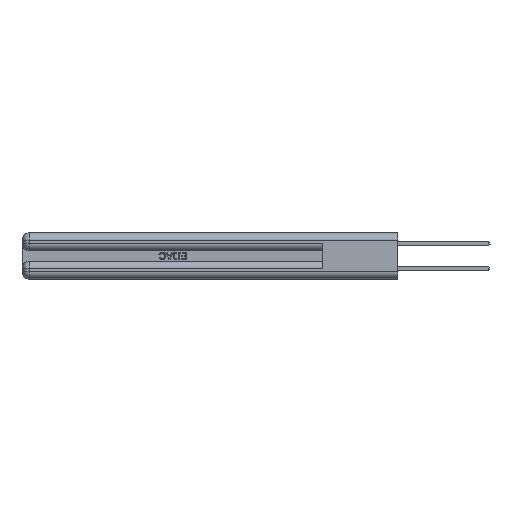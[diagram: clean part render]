
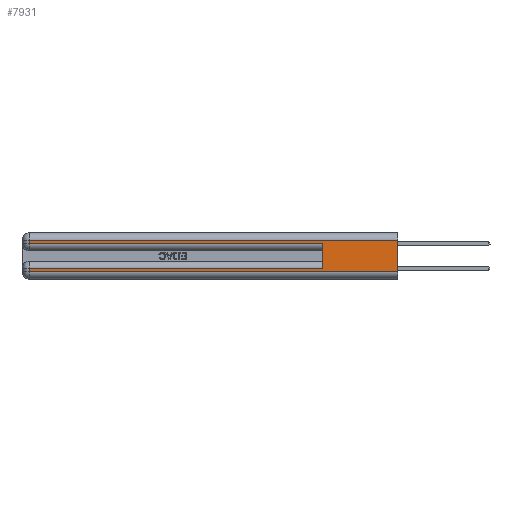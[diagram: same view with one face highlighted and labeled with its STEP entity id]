
A CAD part, left-side view. The second image highlights one B-rep face of the part: STEP entity #7931.
In plain terms, the highlighted planar face has unit normal (-1, 0, 0).
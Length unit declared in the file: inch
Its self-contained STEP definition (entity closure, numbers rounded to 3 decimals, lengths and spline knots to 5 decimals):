
#807 = ORIENTED_EDGE ( 'NONE', *, *, #41067, .T. ) ;
#837 = EDGE_CURVE ( 'NONE', #49698, #30197, #3433, .T. ) ;
#1463 = EDGE_CURVE ( 'NONE', #36310, #22740, #43413, .T. ) ;
#1693 = LINE ( 'NONE', #10921, #42359 ) ;
#2416 = DIRECTION ( 'NONE',  ( 0., -1., 0. ) ) ;
#3433 = LINE ( 'NONE', #16489, #44101 ) ;
#4040 = DIRECTION ( 'NONE',  ( 0., 0., -1. ) ) ;
#4311 = LINE ( 'NONE', #28786, #36922 ) ;
#4662 = AXIS2_PLACEMENT_3D ( 'NONE', #22745, #7198, #34738 ) ;
#4746 = ORIENTED_EDGE ( 'NONE', *, *, #12398, .T. ) ;
#4792 = VERTEX_POINT ( 'NONE', #29184 ) ;
#5282 = DIRECTION ( 'NONE',  ( 0., -1., 0. ) ) ;
#5561 = LINE ( 'NONE', #48295, #34497 ) ;
#7198 = DIRECTION ( 'NONE',  ( 1., 0., 0. ) ) ;
#7931 = ADVANCED_FACE ( 'NONE', ( #9622 ), #30686, .F. ) ;
#8285 = CARTESIAN_POINT ( 'NONE',  ( 0., 0., 0.31 ) ) ;
#9622 = FACE_OUTER_BOUND ( 'NONE', #47696, .T. ) ;
#9890 = CARTESIAN_POINT ( 'NONE',  ( 0., 2.94, 0.285 ) ) ;
#10921 = CARTESIAN_POINT ( 'NONE',  ( 0., 0., 0.37 ) ) ;
#11532 = CARTESIAN_POINT ( 'NONE',  ( 0., 2.94, 0.085 ) ) ;
#11778 = CARTESIAN_POINT ( 'NONE',  ( 0., 2.94, 0.37 ) ) ;
#12398 = EDGE_CURVE ( 'NONE', #28507, #34046, #4311, .T. ) ;
#12491 = CARTESIAN_POINT ( 'NONE',  ( 0., 0.6, 0.145 ) ) ;
#12854 = DIRECTION ( 'NONE',  ( 0., 1., 0. ) ) ;
#16391 = DIRECTION ( 'NONE',  ( 0., 0., 1. ) ) ;
#16489 = CARTESIAN_POINT ( 'NONE',  ( 0., 0., 0.085 ) ) ;
#16516 = VECTOR ( 'NONE', #4040, 39.37008 ) ;
#20144 = ORIENTED_EDGE ( 'NONE', *, *, #837, .T. ) ;
#22740 = VERTEX_POINT ( 'NONE', #41359 ) ;
#22745 = CARTESIAN_POINT ( 'NONE',  ( 0., 0., 0.37 ) ) ;
#23728 = CARTESIAN_POINT ( 'NONE',  ( 0., 0.6, 0.085 ) ) ;
#23778 = ORIENTED_EDGE ( 'NONE', *, *, #37049, .F. ) ;
#25498 = LINE ( 'NONE', #12491, #45324 ) ;
#26975 = LINE ( 'NONE', #11778, #16516 ) ;
#27406 = EDGE_CURVE ( 'NONE', #31264, #4792, #47996, .T. ) ;
#28231 = EDGE_CURVE ( 'NONE', #36310, #34046, #1693, .T. ) ;
#28459 = CARTESIAN_POINT ( 'NONE',  ( 0., 0., 0.31 ) ) ;
#28507 = VERTEX_POINT ( 'NONE', #28527 ) ;
#28527 = CARTESIAN_POINT ( 'NONE',  ( 0., 2.94, 0.06 ) ) ;
#28786 = CARTESIAN_POINT ( 'NONE',  ( 0., 0., 0.06 ) ) ;
#28902 = ORIENTED_EDGE ( 'NONE', *, *, #42451, .T. ) ;
#29184 = CARTESIAN_POINT ( 'NONE',  ( 0., 0.6, 0.285 ) ) ;
#30197 = VERTEX_POINT ( 'NONE', #11532 ) ;
#30293 = ORIENTED_EDGE ( 'NONE', *, *, #28231, .F. ) ;
#30686 = PLANE ( 'NONE',  #4662 ) ;
#31264 = VERTEX_POINT ( 'NONE', #9890 ) ;
#32852 = VECTOR ( 'NONE', #12854, 39.37008 ) ;
#33701 = CARTESIAN_POINT ( 'NONE',  ( 0., 0., 0.06 ) ) ;
#34046 = VERTEX_POINT ( 'NONE', #33701 ) ;
#34497 = VECTOR ( 'NONE', #44167, 39.37008 ) ;
#34738 = DIRECTION ( 'NONE',  ( 0., 0., -1. ) ) ;
#35167 = ORIENTED_EDGE ( 'NONE', *, *, #27406, .T. ) ;
#36310 = VERTEX_POINT ( 'NONE', #8285 ) ;
#36922 = VECTOR ( 'NONE', #5282, 39.37008 ) ;
#37049 = EDGE_CURVE ( 'NONE', #49698, #4792, #25498, .T. ) ;
#37647 = CARTESIAN_POINT ( 'NONE',  ( 0., 0., 0.285 ) ) ;
#40161 = DIRECTION ( 'NONE',  ( 0., 1., 0. ) ) ;
#41067 = EDGE_CURVE ( 'NONE', #30197, #28507, #5561, .T. ) ;
#41359 = CARTESIAN_POINT ( 'NONE',  ( 0., 2.94, 0.31 ) ) ;
#42359 = VECTOR ( 'NONE', #50333, 39.37008 ) ;
#42451 = EDGE_CURVE ( 'NONE', #22740, #31264, #26975, .T. ) ;
#42618 = ORIENTED_EDGE ( 'NONE', *, *, #1463, .T. ) ;
#43413 = LINE ( 'NONE', #28459, #32852 ) ;
#44101 = VECTOR ( 'NONE', #40161, 39.37008 ) ;
#44167 = DIRECTION ( 'NONE',  ( 0., 0., -1. ) ) ;
#45324 = VECTOR ( 'NONE', #16391, 39.37008 ) ;
#46759 = VECTOR ( 'NONE', #2416, 39.37008 ) ;
#47696 = EDGE_LOOP ( 'NONE', ( #30293, #42618, #28902, #35167, #23778, #20144, #807, #4746 ) ) ;
#47996 = LINE ( 'NONE', #37647, #46759 ) ;
#48295 = CARTESIAN_POINT ( 'NONE',  ( 0., 2.94, 0.37 ) ) ;
#49698 = VERTEX_POINT ( 'NONE', #23728 ) ;
#50333 = DIRECTION ( 'NONE',  ( 0., 0., -1. ) ) ;
